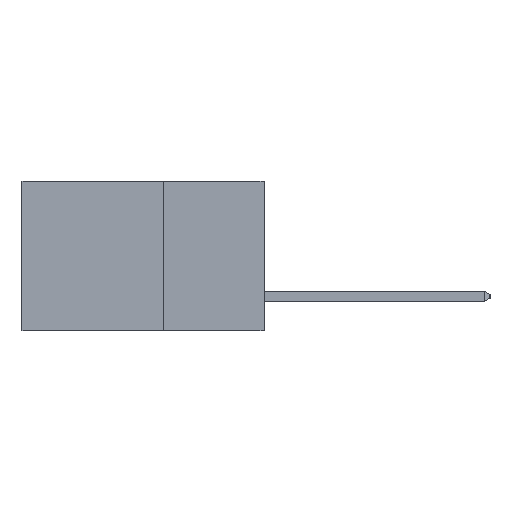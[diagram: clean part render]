
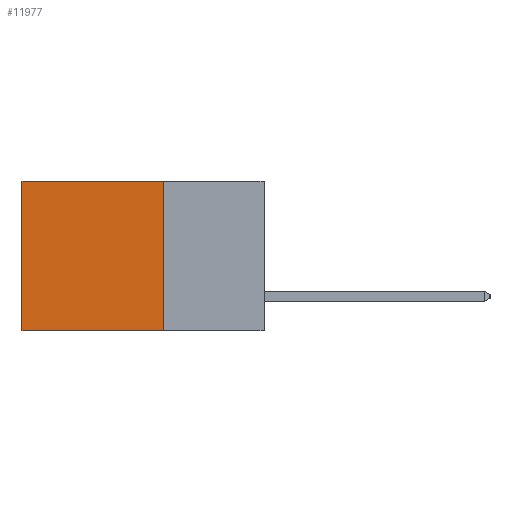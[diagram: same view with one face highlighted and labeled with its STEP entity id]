
A CAD part, left-side view. The second image highlights one B-rep face of the part: STEP entity #11977.
In plain terms, the highlighted planar face has unit normal (-1, 0, 0).
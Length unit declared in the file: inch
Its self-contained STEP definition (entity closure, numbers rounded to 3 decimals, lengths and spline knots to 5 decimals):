
#460 = ORIENTED_EDGE ( 'NONE', *, *, #1932, .F. ) ;
#498 = ORIENTED_EDGE ( 'NONE', *, *, #17240, .T. ) ;
#1932 = EDGE_CURVE ( 'NONE', #20565, #5336, #11418, .T. ) ;
#2542 = CARTESIAN_POINT ( 'NONE',  ( 0.2615, 0.6, 0. ) ) ;
#2712 = PLANE ( 'NONE',  #7835 ) ;
#3416 = CARTESIAN_POINT ( 'NONE',  ( 0.2615, 0.25, -0.37 ) ) ;
#3421 = EDGE_CURVE ( 'NONE', #5336, #11545, #5073, .T. ) ;
#3710 = CARTESIAN_POINT ( 'NONE',  ( 0.2615, 0.25, 0. ) ) ;
#3774 = DIRECTION ( 'NONE',  ( 0., 1., 0. ) ) ;
#5073 = LINE ( 'NONE', #15850, #17244 ) ;
#5336 = VERTEX_POINT ( 'NONE', #3416 ) ;
#5631 = VECTOR ( 'NONE', #3774, 39.37008 ) ;
#5976 = CARTESIAN_POINT ( 'NONE',  ( 0.2615, 0.25, -0.37 ) ) ;
#6753 = ORIENTED_EDGE ( 'NONE', *, *, #3421, .F. ) ;
#7152 = VECTOR ( 'NONE', #11749, 39.37008 ) ;
#7615 = DIRECTION ( 'NONE',  ( 0., 0., -1. ) ) ;
#7835 = AXIS2_PLACEMENT_3D ( 'NONE', #5976, #17090, #7615 ) ;
#10414 = EDGE_CURVE ( 'NONE', #20565, #18034, #13635, .T. ) ;
#10768 = FACE_OUTER_BOUND ( 'NONE', #13980, .T. ) ;
#11418 = LINE ( 'NONE', #11696, #7152 ) ;
#11545 = VERTEX_POINT ( 'NONE', #20622 ) ;
#11696 = CARTESIAN_POINT ( 'NONE',  ( 0.2615, 0.25, -0.37 ) ) ;
#11749 = DIRECTION ( 'NONE',  ( 0., 0., -1. ) ) ;
#11977 = ADVANCED_FACE ( 'NONE', ( #10768 ), #2712, .F. ) ;
#12501 = LINE ( 'NONE', #15660, #16660 ) ;
#12518 = DIRECTION ( 'NONE',  ( 0., 0., -1. ) ) ;
#13635 = LINE ( 'NONE', #14930, #5631 ) ;
#13980 = EDGE_LOOP ( 'NONE', ( #498, #6753, #460, #17413 ) ) ;
#14795 = DIRECTION ( 'NONE',  ( 0., 1., 0. ) ) ;
#14930 = CARTESIAN_POINT ( 'NONE',  ( 0.2615, 0.25, 0. ) ) ;
#15660 = CARTESIAN_POINT ( 'NONE',  ( 0.2615, 0.6, -0.37 ) ) ;
#15850 = CARTESIAN_POINT ( 'NONE',  ( 0.2615, 0.25, -0.37 ) ) ;
#16660 = VECTOR ( 'NONE', #12518, 39.37008 ) ;
#17090 = DIRECTION ( 'NONE',  ( 1., 0., 0. ) ) ;
#17240 = EDGE_CURVE ( 'NONE', #18034, #11545, #12501, .T. ) ;
#17244 = VECTOR ( 'NONE', #14795, 39.37008 ) ;
#17413 = ORIENTED_EDGE ( 'NONE', *, *, #10414, .T. ) ;
#18034 = VERTEX_POINT ( 'NONE', #2542 ) ;
#20565 = VERTEX_POINT ( 'NONE', #3710 ) ;
#20622 = CARTESIAN_POINT ( 'NONE',  ( 0.2615, 0.6, -0.37 ) ) ;
